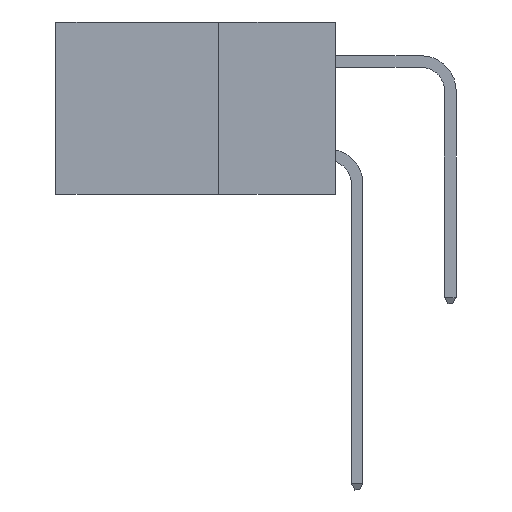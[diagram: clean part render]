
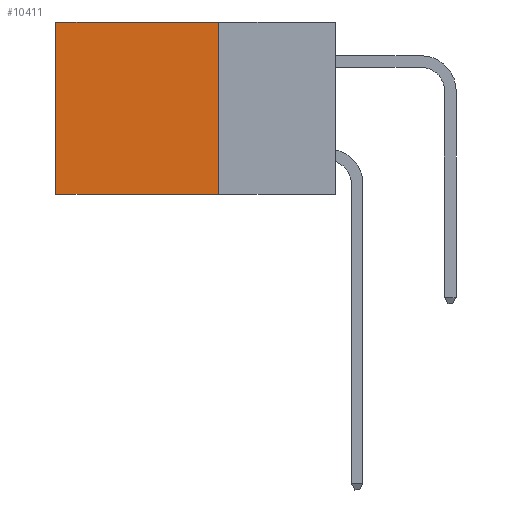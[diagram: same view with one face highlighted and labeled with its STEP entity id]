
A CAD part, left-side view. The second image highlights one B-rep face of the part: STEP entity #10411.
In plain terms, the highlighted planar face has unit normal (-1, 0, 0).
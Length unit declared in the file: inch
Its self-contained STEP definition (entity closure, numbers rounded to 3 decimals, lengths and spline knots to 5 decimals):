
#1173 = LINE ( 'NONE', #20338, #12407 ) ;
#3349 = CARTESIAN_POINT ( 'NONE',  ( 0.2875, 0.25, -0.37 ) ) ;
#4271 = VERTEX_POINT ( 'NONE', #18042 ) ;
#4539 = EDGE_CURVE ( 'NONE', #5424, #12927, #15957, .T. ) ;
#4929 = ORIENTED_EDGE ( 'NONE', *, *, #10422, .F. ) ;
#5424 = VERTEX_POINT ( 'NONE', #17087 ) ;
#6387 = CARTESIAN_POINT ( 'NONE',  ( 0.2875, 0.25, 0. ) ) ;
#7560 = CARTESIAN_POINT ( 'NONE',  ( 0.2875, 0.6, -0.37 ) ) ;
#7768 = DIRECTION ( 'NONE',  ( 0., 0., -1. ) ) ;
#8332 = EDGE_LOOP ( 'NONE', ( #12200, #4929, #10526, #12901 ) ) ;
#10260 = FACE_OUTER_BOUND ( 'NONE', #8332, .T. ) ;
#10411 = ADVANCED_FACE ( 'NONE', ( #10260 ), #21578, .F. ) ;
#10422 = EDGE_CURVE ( 'NONE', #12927, #18400, #26900, .T. ) ;
#10526 = ORIENTED_EDGE ( 'NONE', *, *, #4539, .F. ) ;
#10659 = CARTESIAN_POINT ( 'NONE',  ( 0.2875, 0.25, -0.37 ) ) ;
#10932 = DIRECTION ( 'NONE',  ( 0., 0., -1. ) ) ;
#12200 = ORIENTED_EDGE ( 'NONE', *, *, #27293, .T. ) ;
#12407 = VECTOR ( 'NONE', #16202, 39.37008 ) ;
#12901 = ORIENTED_EDGE ( 'NONE', *, *, #25969, .T. ) ;
#12927 = VERTEX_POINT ( 'NONE', #3349 ) ;
#15321 = VECTOR ( 'NONE', #25772, 39.37008 ) ;
#15660 = VECTOR ( 'NONE', #7768, 39.37008 ) ;
#15957 = LINE ( 'NONE', #6387, #26873 ) ;
#16202 = DIRECTION ( 'NONE',  ( 0., 1., 0. ) ) ;
#16442 = AXIS2_PLACEMENT_3D ( 'NONE', #28048, #27958, #10932 ) ;
#17087 = CARTESIAN_POINT ( 'NONE',  ( 0.2875, 0.25, 0. ) ) ;
#17725 = LINE ( 'NONE', #23345, #15660 ) ;
#18042 = CARTESIAN_POINT ( 'NONE',  ( 0.2875, 0.6, 0. ) ) ;
#18400 = VERTEX_POINT ( 'NONE', #7560 ) ;
#20338 = CARTESIAN_POINT ( 'NONE',  ( 0.2875, 0.25, 0. ) ) ;
#21578 = PLANE ( 'NONE',  #16442 ) ;
#23345 = CARTESIAN_POINT ( 'NONE',  ( 0.2875, 0.6, 0. ) ) ;
#25772 = DIRECTION ( 'NONE',  ( 0., 1., 0. ) ) ;
#25969 = EDGE_CURVE ( 'NONE', #5424, #4271, #1173, .T. ) ;
#26873 = VECTOR ( 'NONE', #28060, 39.37008 ) ;
#26900 = LINE ( 'NONE', #10659, #15321 ) ;
#27293 = EDGE_CURVE ( 'NONE', #4271, #18400, #17725, .T. ) ;
#27958 = DIRECTION ( 'NONE',  ( 1., 0., 0. ) ) ;
#28048 = CARTESIAN_POINT ( 'NONE',  ( 0.2875, 0.25, 0. ) ) ;
#28060 = DIRECTION ( 'NONE',  ( 0., 0., -1. ) ) ;
